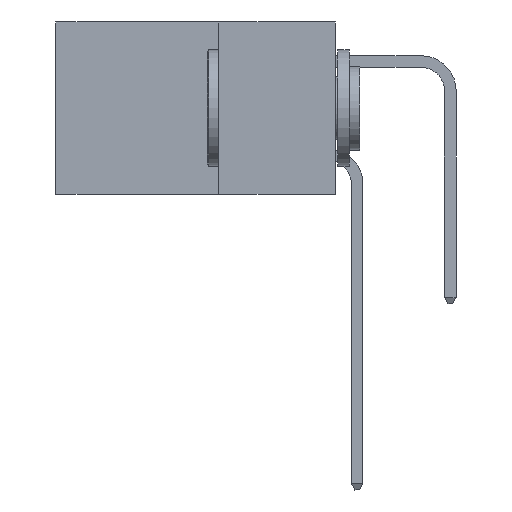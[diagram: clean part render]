
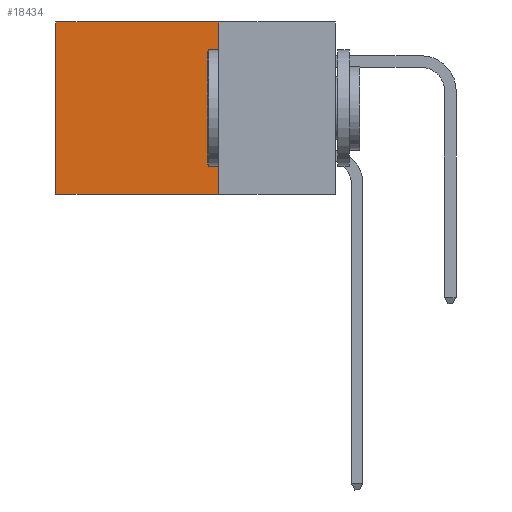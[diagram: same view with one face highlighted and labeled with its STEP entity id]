
A CAD part, left-side view. The second image highlights one B-rep face of the part: STEP entity #18434.
In plain terms, the highlighted planar face has unit normal (-1, 0, 0).
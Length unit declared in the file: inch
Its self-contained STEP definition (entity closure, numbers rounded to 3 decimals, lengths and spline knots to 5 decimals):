
#24 = LINE ( 'NONE', #12649, #11711 ) ;
#255 = EDGE_LOOP ( 'NONE', ( #15002, #7448, #8914, #6630 ) ) ;
#675 = DIRECTION ( 'NONE',  ( 0., 0., -1. ) ) ;
#932 = DIRECTION ( 'NONE',  ( 0., 1., 0. ) ) ;
#1821 = VECTOR ( 'NONE', #8768, 39.37008 ) ;
#1991 = VECTOR ( 'NONE', #932, 39.37008 ) ;
#3515 = EDGE_CURVE ( 'NONE', #12820, #12139, #24, .T. ) ;
#3864 = EDGE_CURVE ( 'NONE', #12139, #10616, #3875, .T. ) ;
#3875 = LINE ( 'NONE', #10307, #1821 ) ;
#5029 = FACE_OUTER_BOUND ( 'NONE', #255, .T. ) ;
#6630 = ORIENTED_EDGE ( 'NONE', *, *, #11415, .T. ) ;
#7448 = ORIENTED_EDGE ( 'NONE', *, *, #3864, .F. ) ;
#7613 = DIRECTION ( 'NONE',  ( 1., 0., 0. ) ) ;
#7979 = CARTESIAN_POINT ( 'NONE',  ( 0.2875, 0.6, 0. ) ) ;
#8768 = DIRECTION ( 'NONE',  ( 0., 1., 0. ) ) ;
#8914 = ORIENTED_EDGE ( 'NONE', *, *, #3515, .F. ) ;
#9748 = DIRECTION ( 'NONE',  ( 0., 0., -1. ) ) ;
#10307 = CARTESIAN_POINT ( 'NONE',  ( 0.2875, 0.25, -0.37 ) ) ;
#10616 = VERTEX_POINT ( 'NONE', #17114 ) ;
#11415 = EDGE_CURVE ( 'NONE', #12820, #21475, #15838, .T. ) ;
#11711 = VECTOR ( 'NONE', #675, 39.37008 ) ;
#12139 = VERTEX_POINT ( 'NONE', #18805 ) ;
#12649 = CARTESIAN_POINT ( 'NONE',  ( 0.2875, 0.25, 0. ) ) ;
#12707 = CARTESIAN_POINT ( 'NONE',  ( 0.2875, 0.25, 0. ) ) ;
#12782 = PLANE ( 'NONE',  #18008 ) ;
#12820 = VERTEX_POINT ( 'NONE', #13420 ) ;
#13210 = EDGE_CURVE ( 'NONE', #21475, #10616, #13369, .T. ) ;
#13369 = LINE ( 'NONE', #18016, #16289 ) ;
#13420 = CARTESIAN_POINT ( 'NONE',  ( 0.2875, 0.25, 0. ) ) ;
#14023 = CARTESIAN_POINT ( 'NONE',  ( 0.2875, 0.25, 0. ) ) ;
#15002 = ORIENTED_EDGE ( 'NONE', *, *, #13210, .T. ) ;
#15838 = LINE ( 'NONE', #14023, #1991 ) ;
#16289 = VECTOR ( 'NONE', #9748, 39.37008 ) ;
#17114 = CARTESIAN_POINT ( 'NONE',  ( 0.2875, 0.6, -0.37 ) ) ;
#17985 = DIRECTION ( 'NONE',  ( 0., 0., -1. ) ) ;
#18008 = AXIS2_PLACEMENT_3D ( 'NONE', #12707, #7613, #17985 ) ;
#18016 = CARTESIAN_POINT ( 'NONE',  ( 0.2875, 0.6, 0. ) ) ;
#18434 = ADVANCED_FACE ( 'NONE', ( #5029 ), #12782, .F. ) ;
#18805 = CARTESIAN_POINT ( 'NONE',  ( 0.2875, 0.25, -0.37 ) ) ;
#21475 = VERTEX_POINT ( 'NONE', #7979 ) ;
